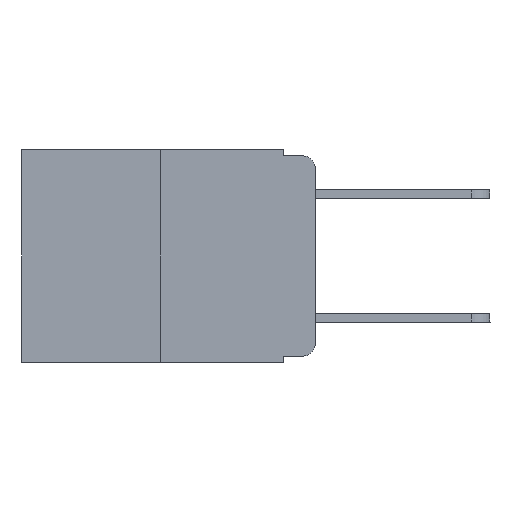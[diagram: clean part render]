
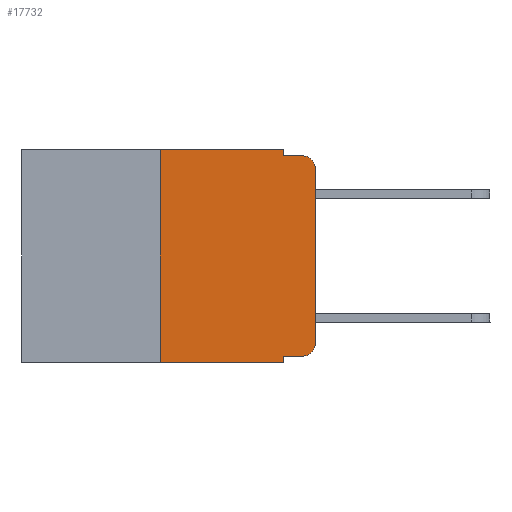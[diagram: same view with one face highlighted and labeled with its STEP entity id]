
A CAD part, left-side view. The second image highlights one B-rep face of the part: STEP entity #17732.
In plain terms, the highlighted planar face has unit normal (-1, 0, 0).
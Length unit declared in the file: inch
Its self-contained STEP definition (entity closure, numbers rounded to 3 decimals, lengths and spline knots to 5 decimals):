
#225 = LINE ( 'NONE', #15156, #14889 ) ;
#527 = VECTOR ( 'NONE', #17566, 39.37008 ) ;
#1271 = DIRECTION ( 'NONE',  ( 0., -1., 0. ) ) ;
#1383 = AXIS2_PLACEMENT_3D ( 'NONE', #7629, #13284, #17632 ) ;
#1489 = VERTEX_POINT ( 'NONE', #9471 ) ;
#1719 = VECTOR ( 'NONE', #6466, 39.37008 ) ;
#1721 = ORIENTED_EDGE ( 'NONE', *, *, #1941, .T. ) ;
#1941 = EDGE_CURVE ( 'NONE', #6400, #12950, #9855, .T. ) ;
#2246 = VERTEX_POINT ( 'NONE', #24206 ) ;
#2391 = VERTEX_POINT ( 'NONE', #22997 ) ;
#2674 = VERTEX_POINT ( 'NONE', #7155 ) ;
#2925 = CARTESIAN_POINT ( 'NONE',  ( 0., 0., 0. ) ) ;
#3311 = DIRECTION ( 'NONE',  ( -1., 0., 0. ) ) ;
#4360 = DIRECTION ( 'NONE',  ( 0., 0., -1. ) ) ;
#4422 = EDGE_LOOP ( 'NONE', ( #14217, #1721, #8222, #23168, #5152, #22299, #8910, #20482, #6610, #8618 ) ) ;
#4426 = CARTESIAN_POINT ( 'NONE',  ( 0., 0.02, -0.01 ) ) ;
#4729 = CARTESIAN_POINT ( 'NONE',  ( 0., 0.25, 0. ) ) ;
#4937 = CARTESIAN_POINT ( 'NONE',  ( 0., 0.051, -0.333 ) ) ;
#5140 = CARTESIAN_POINT ( 'NONE',  ( 0., 0., -0.03 ) ) ;
#5152 = ORIENTED_EDGE ( 'NONE', *, *, #10945, .F. ) ;
#5443 = CARTESIAN_POINT ( 'NONE',  ( 0., 0.051, -0.01 ) ) ;
#6077 = LINE ( 'NONE', #5443, #23154 ) ;
#6226 = EDGE_CURVE ( 'NONE', #8348, #20810, #17526, .T. ) ;
#6260 = VECTOR ( 'NONE', #4360, 39.37008 ) ;
#6376 = DIRECTION ( 'NONE',  ( 0., 0., -1. ) ) ;
#6400 = VERTEX_POINT ( 'NONE', #5140 ) ;
#6456 = EDGE_CURVE ( 'NONE', #15601, #6400, #13412, .T. ) ;
#6463 = CARTESIAN_POINT ( 'NONE',  ( 0., 0.02, -0.03 ) ) ;
#6466 = DIRECTION ( 'NONE',  ( 0., 0., 1. ) ) ;
#6610 = ORIENTED_EDGE ( 'NONE', *, *, #16661, .T. ) ;
#6996 = AXIS2_PLACEMENT_3D ( 'NONE', #18785, #3311, #7517 ) ;
#7155 = CARTESIAN_POINT ( 'NONE',  ( 0., 0.25, 0. ) ) ;
#7517 = DIRECTION ( 'NONE',  ( 0., 0., -1. ) ) ;
#7629 = CARTESIAN_POINT ( 'NONE',  ( 0., 0.473, 0. ) ) ;
#8222 = ORIENTED_EDGE ( 'NONE', *, *, #20207, .F. ) ;
#8348 = VERTEX_POINT ( 'NONE', #23548 ) ;
#8618 = ORIENTED_EDGE ( 'NONE', *, *, #23472, .T. ) ;
#8910 = ORIENTED_EDGE ( 'NONE', *, *, #22193, .T. ) ;
#9383 = VECTOR ( 'NONE', #10792, 39.37008 ) ;
#9471 = CARTESIAN_POINT ( 'NONE',  ( 0., 0.051, 0. ) ) ;
#9822 = CIRCLE ( 'NONE', #6996, 0.02 ) ;
#9855 = CIRCLE ( 'NONE', #14960, 0.02 ) ;
#10018 = CARTESIAN_POINT ( 'NONE',  ( 0., 0.051, 0. ) ) ;
#10792 = DIRECTION ( 'NONE',  ( 0., -1., 0. ) ) ;
#10945 = EDGE_CURVE ( 'NONE', #2674, #1489, #19137, .T. ) ;
#11561 = FACE_OUTER_BOUND ( 'NONE', #4422, .T. ) ;
#12041 = EDGE_CURVE ( 'NONE', #20397, #2674, #12911, .T. ) ;
#12617 = CARTESIAN_POINT ( 'NONE',  ( 0., 0.473, 0. ) ) ;
#12869 = DIRECTION ( 'NONE',  ( 0., -1., 0. ) ) ;
#12911 = LINE ( 'NONE', #4729, #1719 ) ;
#12950 = VERTEX_POINT ( 'NONE', #4426 ) ;
#12985 = CARTESIAN_POINT ( 'NONE',  ( 0., 0., -0.313 ) ) ;
#13284 = DIRECTION ( 'NONE',  ( 1., 0., 0. ) ) ;
#13412 = LINE ( 'NONE', #2925, #19315 ) ;
#13444 = EDGE_CURVE ( 'NONE', #1489, #2246, #18928, .T. ) ;
#14039 = CARTESIAN_POINT ( 'NONE',  ( 0., 0.051, 0. ) ) ;
#14217 = ORIENTED_EDGE ( 'NONE', *, *, #6456, .T. ) ;
#14889 = VECTOR ( 'NONE', #15244, 39.37008 ) ;
#14960 = AXIS2_PLACEMENT_3D ( 'NONE', #6463, #19402, #6376 ) ;
#15156 = CARTESIAN_POINT ( 'NONE',  ( 0., 0.473, -0.343 ) ) ;
#15244 = DIRECTION ( 'NONE',  ( 0., -1., 0. ) ) ;
#15601 = VERTEX_POINT ( 'NONE', #12985 ) ;
#16068 = DIRECTION ( 'NONE',  ( 0., 0., 1. ) ) ;
#16661 = EDGE_CURVE ( 'NONE', #8348, #2391, #17753, .T. ) ;
#17526 = LINE ( 'NONE', #14039, #527 ) ;
#17566 = DIRECTION ( 'NONE',  ( 0., 0., -1. ) ) ;
#17632 = DIRECTION ( 'NONE',  ( 0., 0., -1. ) ) ;
#17732 = ADVANCED_FACE ( 'NONE', ( #11561 ), #18888, .F. ) ;
#17753 = LINE ( 'NONE', #4937, #21607 ) ;
#18250 = CARTESIAN_POINT ( 'NONE',  ( 0., 0.051, -0.343 ) ) ;
#18777 = CARTESIAN_POINT ( 'NONE',  ( 0., 0.25, -0.343 ) ) ;
#18785 = CARTESIAN_POINT ( 'NONE',  ( 0., 0.02, -0.313 ) ) ;
#18888 = PLANE ( 'NONE',  #1383 ) ;
#18928 = LINE ( 'NONE', #10018, #6260 ) ;
#19137 = LINE ( 'NONE', #12617, #9383 ) ;
#19315 = VECTOR ( 'NONE', #16068, 39.37008 ) ;
#19402 = DIRECTION ( 'NONE',  ( -1., 0., 0. ) ) ;
#20207 = EDGE_CURVE ( 'NONE', #2246, #12950, #6077, .T. ) ;
#20397 = VERTEX_POINT ( 'NONE', #18777 ) ;
#20482 = ORIENTED_EDGE ( 'NONE', *, *, #6226, .F. ) ;
#20810 = VERTEX_POINT ( 'NONE', #18250 ) ;
#21607 = VECTOR ( 'NONE', #1271, 39.37008 ) ;
#22193 = EDGE_CURVE ( 'NONE', #20397, #20810, #225, .T. ) ;
#22299 = ORIENTED_EDGE ( 'NONE', *, *, #12041, .F. ) ;
#22997 = CARTESIAN_POINT ( 'NONE',  ( 0., 0.02, -0.333 ) ) ;
#23154 = VECTOR ( 'NONE', #12869, 39.37008 ) ;
#23168 = ORIENTED_EDGE ( 'NONE', *, *, #13444, .F. ) ;
#23472 = EDGE_CURVE ( 'NONE', #2391, #15601, #9822, .T. ) ;
#23548 = CARTESIAN_POINT ( 'NONE',  ( 0., 0.051, -0.333 ) ) ;
#24206 = CARTESIAN_POINT ( 'NONE',  ( 0., 0.051, -0.01 ) ) ;
